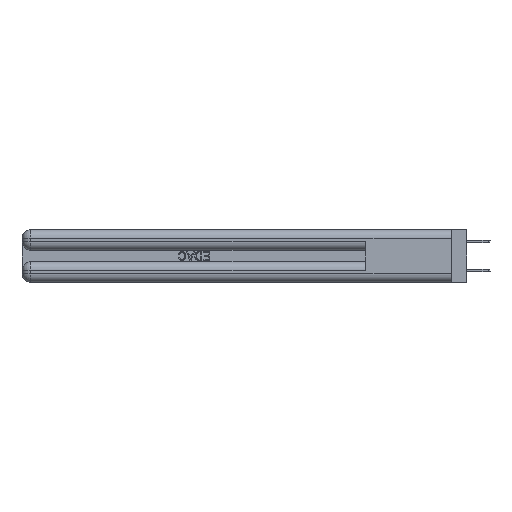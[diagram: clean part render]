
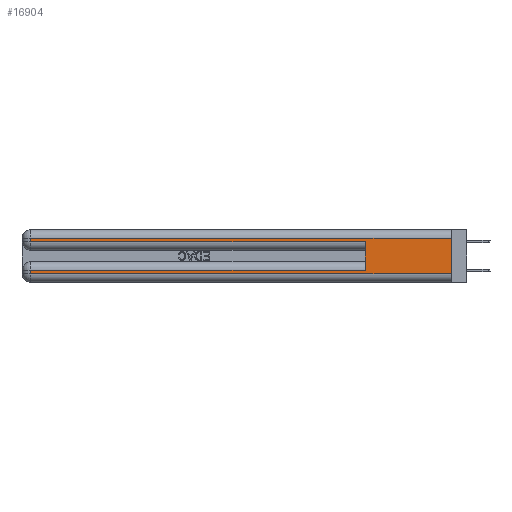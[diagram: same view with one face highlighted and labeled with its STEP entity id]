
A CAD part, left-side view. The second image highlights one B-rep face of the part: STEP entity #16904.
In plain terms, the highlighted planar face has unit normal (-1, 0, 0).
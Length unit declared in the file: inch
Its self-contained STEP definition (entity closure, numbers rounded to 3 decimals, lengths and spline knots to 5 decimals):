
#384 = ORIENTED_EDGE ( 'NONE', *, *, #9772, .T. ) ;
#1704 = CARTESIAN_POINT ( 'NONE',  ( 0., 0., 0.37 ) ) ;
#1960 = VERTEX_POINT ( 'NONE', #19528 ) ;
#2519 = ORIENTED_EDGE ( 'NONE', *, *, #16267, .F. ) ;
#2539 = ORIENTED_EDGE ( 'NONE', *, *, #24889, .T. ) ;
#2575 = VECTOR ( 'NONE', #5892, 39.37008 ) ;
#2655 = VERTEX_POINT ( 'NONE', #7789 ) ;
#2809 = VECTOR ( 'NONE', #10716, 39.37008 ) ;
#2832 = CARTESIAN_POINT ( 'NONE',  ( 0., 0., 0.085 ) ) ;
#2877 = LINE ( 'NONE', #1704, #25688 ) ;
#3369 = CARTESIAN_POINT ( 'NONE',  ( 0., 2.94, 0.06 ) ) ;
#3576 = ORIENTED_EDGE ( 'NONE', *, *, #29513, .T. ) ;
#4268 = FACE_OUTER_BOUND ( 'NONE', #6764, .T. ) ;
#4581 = ORIENTED_EDGE ( 'NONE', *, *, #4933, .F. ) ;
#4650 = CARTESIAN_POINT ( 'NONE',  ( 0., 0., 0.31 ) ) ;
#4933 = EDGE_CURVE ( 'NONE', #37312, #6401, #23505, .T. ) ;
#5892 = DIRECTION ( 'NONE',  ( 0., 1., 0. ) ) ;
#6016 = DIRECTION ( 'NONE',  ( 0., -1., 0. ) ) ;
#6401 = VERTEX_POINT ( 'NONE', #9753 ) ;
#6614 = ORIENTED_EDGE ( 'NONE', *, *, #30717, .T. ) ;
#6764 = EDGE_LOOP ( 'NONE', ( #2519, #6614, #2539, #10360, #4581, #3576, #384, #12136 ) ) ;
#6846 = VERTEX_POINT ( 'NONE', #32571 ) ;
#7455 = AXIS2_PLACEMENT_3D ( 'NONE', #7799, #28963, #11363 ) ;
#7735 = EDGE_CURVE ( 'NONE', #20209, #6846, #26547, .T. ) ;
#7789 = CARTESIAN_POINT ( 'NONE',  ( 0., 2.94, 0.085 ) ) ;
#7799 = CARTESIAN_POINT ( 'NONE',  ( 0., 0., 0.37 ) ) ;
#9021 = CARTESIAN_POINT ( 'NONE',  ( 0., 2.94, 0.37 ) ) ;
#9044 = VERTEX_POINT ( 'NONE', #9919 ) ;
#9709 = LINE ( 'NONE', #2832, #2575 ) ;
#9753 = CARTESIAN_POINT ( 'NONE',  ( 0., 0.6, 0.285 ) ) ;
#9772 = EDGE_CURVE ( 'NONE', #2655, #20209, #13081, .T. ) ;
#9919 = CARTESIAN_POINT ( 'NONE',  ( 0., 0., 0.31 ) ) ;
#10360 = ORIENTED_EDGE ( 'NONE', *, *, #13063, .T. ) ;
#10716 = DIRECTION ( 'NONE',  ( 0., -1., 0. ) ) ;
#11161 = LINE ( 'NONE', #29692, #25899 ) ;
#11363 = DIRECTION ( 'NONE',  ( 0., 0., -1. ) ) ;
#12062 = VECTOR ( 'NONE', #37011, 39.37008 ) ;
#12083 = DIRECTION ( 'NONE',  ( 0., 0., -1. ) ) ;
#12136 = ORIENTED_EDGE ( 'NONE', *, *, #7735, .T. ) ;
#12993 = LINE ( 'NONE', #4650, #12062 ) ;
#13063 = EDGE_CURVE ( 'NONE', #1960, #6401, #11161, .T. ) ;
#13081 = LINE ( 'NONE', #19327, #35504 ) ;
#13237 = CARTESIAN_POINT ( 'NONE',  ( 0., 0.6, 0.085 ) ) ;
#13714 = CARTESIAN_POINT ( 'NONE',  ( 0., 0., 0.06 ) ) ;
#14867 = VERTEX_POINT ( 'NONE', #29061 ) ;
#16267 = EDGE_CURVE ( 'NONE', #9044, #6846, #2877, .T. ) ;
#16904 = ADVANCED_FACE ( 'NONE', ( #4268 ), #25531, .F. ) ;
#17471 = CARTESIAN_POINT ( 'NONE',  ( 0., 0.6, 0.145 ) ) ;
#19327 = CARTESIAN_POINT ( 'NONE',  ( 0., 2.94, 0.37 ) ) ;
#19528 = CARTESIAN_POINT ( 'NONE',  ( 0., 2.94, 0.285 ) ) ;
#20209 = VERTEX_POINT ( 'NONE', #3369 ) ;
#22052 = LINE ( 'NONE', #9021, #28900 ) ;
#22478 = DIRECTION ( 'NONE',  ( 0., 0., -1. ) ) ;
#23505 = LINE ( 'NONE', #17471, #30349 ) ;
#24889 = EDGE_CURVE ( 'NONE', #14867, #1960, #22052, .T. ) ;
#25531 = PLANE ( 'NONE',  #7455 ) ;
#25688 = VECTOR ( 'NONE', #22478, 39.37008 ) ;
#25899 = VECTOR ( 'NONE', #6016, 39.37008 ) ;
#26547 = LINE ( 'NONE', #13714, #2809 ) ;
#28900 = VECTOR ( 'NONE', #12083, 39.37008 ) ;
#28963 = DIRECTION ( 'NONE',  ( 1., 0., 0. ) ) ;
#29061 = CARTESIAN_POINT ( 'NONE',  ( 0., 2.94, 0.31 ) ) ;
#29513 = EDGE_CURVE ( 'NONE', #37312, #2655, #9709, .T. ) ;
#29692 = CARTESIAN_POINT ( 'NONE',  ( 0., 0., 0.285 ) ) ;
#30349 = VECTOR ( 'NONE', #34986, 39.37008 ) ;
#30717 = EDGE_CURVE ( 'NONE', #9044, #14867, #12993, .T. ) ;
#31075 = DIRECTION ( 'NONE',  ( 0., 0., -1. ) ) ;
#32571 = CARTESIAN_POINT ( 'NONE',  ( 0., 0., 0.06 ) ) ;
#34986 = DIRECTION ( 'NONE',  ( 0., 0., 1. ) ) ;
#35504 = VECTOR ( 'NONE', #31075, 39.37008 ) ;
#37011 = DIRECTION ( 'NONE',  ( 0., 1., 0. ) ) ;
#37312 = VERTEX_POINT ( 'NONE', #13237 ) ;
